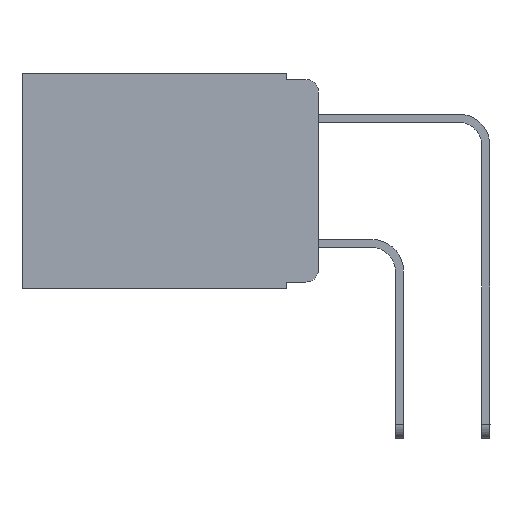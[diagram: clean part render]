
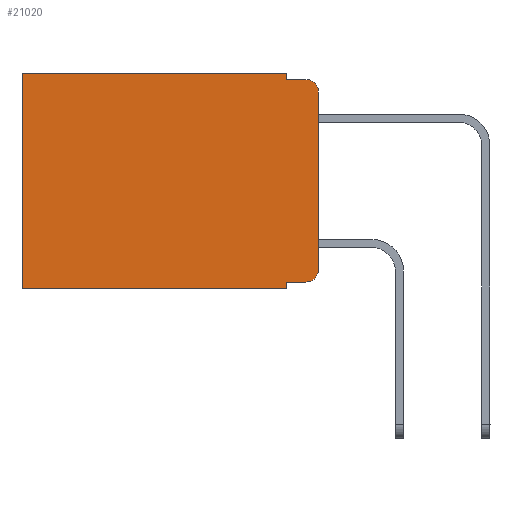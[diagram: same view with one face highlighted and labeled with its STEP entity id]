
A CAD part, left-side view. The second image highlights one B-rep face of the part: STEP entity #21020.
In plain terms, the highlighted planar face has unit normal (-1, 0, 0).
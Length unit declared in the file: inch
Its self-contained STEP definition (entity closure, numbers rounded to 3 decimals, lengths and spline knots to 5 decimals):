
#37 = VECTOR ( 'NONE', #13561, 39.37008 ) ;
#438 = DIRECTION ( 'NONE',  ( 0., 1., 0. ) ) ;
#453 = CARTESIAN_POINT ( 'NONE',  ( 0.298, 0., -0.343 ) ) ;
#503 = ORIENTED_EDGE ( 'NONE', *, *, #20893, .F. ) ;
#535 = CARTESIAN_POINT ( 'NONE',  ( 0.298, 0., 0. ) ) ;
#558 = DIRECTION ( 'NONE',  ( 0., 0., -1. ) ) ;
#646 = DIRECTION ( 'NONE',  ( -1., 0., 0. ) ) ;
#1239 = CARTESIAN_POINT ( 'NONE',  ( 0.298, 0.051, 0. ) ) ;
#1347 = VERTEX_POINT ( 'NONE', #8051 ) ;
#1409 = ORIENTED_EDGE ( 'NONE', *, *, #9598, .F. ) ;
#1495 = CARTESIAN_POINT ( 'NONE',  ( 0.298, 0.02, -0.03 ) ) ;
#1526 = DIRECTION ( 'NONE',  ( 0., 0., -1. ) ) ;
#1839 = AXIS2_PLACEMENT_3D ( 'NONE', #535, #12584, #7223 ) ;
#1972 = CARTESIAN_POINT ( 'NONE',  ( 0.298, 0., 0. ) ) ;
#2070 = PLANE ( 'NONE',  #1839 ) ;
#2104 = EDGE_CURVE ( 'NONE', #11948, #15427, #5297, .T. ) ;
#2612 = VERTEX_POINT ( 'NONE', #21435 ) ;
#3459 = DIRECTION ( 'NONE',  ( 0., -1., 0. ) ) ;
#3470 = ORIENTED_EDGE ( 'NONE', *, *, #9523, .F. ) ;
#3504 = ORIENTED_EDGE ( 'NONE', *, *, #13205, .T. ) ;
#3536 = VECTOR ( 'NONE', #438, 39.37008 ) ;
#3692 = VERTEX_POINT ( 'NONE', #17944 ) ;
#4054 = ORIENTED_EDGE ( 'NONE', *, *, #5171, .F. ) ;
#4130 = CARTESIAN_POINT ( 'NONE',  ( 0.298, 0., -0.03 ) ) ;
#5079 = CARTESIAN_POINT ( 'NONE',  ( 0.298, 0.051, -0.343 ) ) ;
#5171 = EDGE_CURVE ( 'NONE', #1347, #13884, #13077, .T. ) ;
#5297 = CIRCLE ( 'NONE', #17579, 0.02 ) ;
#5930 = CARTESIAN_POINT ( 'NONE',  ( 0.298, 0.02, -0.01 ) ) ;
#6796 = LINE ( 'NONE', #1972, #3536 ) ;
#6936 = VECTOR ( 'NONE', #558, 39.37008 ) ;
#7045 = ORIENTED_EDGE ( 'NONE', *, *, #19641, .F. ) ;
#7223 = DIRECTION ( 'NONE',  ( 0., 0., -1. ) ) ;
#7253 = LINE ( 'NONE', #20646, #6936 ) ;
#7352 = DIRECTION ( 'NONE',  ( 0., 0., -1. ) ) ;
#7904 = VERTEX_POINT ( 'NONE', #18206 ) ;
#8051 = CARTESIAN_POINT ( 'NONE',  ( 0.298, 0.051, -0.333 ) ) ;
#8715 = VERTEX_POINT ( 'NONE', #4130 ) ;
#9043 = EDGE_CURVE ( 'NONE', #1347, #11948, #18480, .T. ) ;
#9523 = EDGE_CURVE ( 'NONE', #8715, #15427, #7253, .T. ) ;
#9598 = EDGE_CURVE ( 'NONE', #13884, #11979, #20423, .T. ) ;
#9652 = VERTEX_POINT ( 'NONE', #5930 ) ;
#10512 = CIRCLE ( 'NONE', #15761, 0.02 ) ;
#11040 = EDGE_CURVE ( 'NONE', #2612, #11979, #18216, .T. ) ;
#11823 = LINE ( 'NONE', #15349, #17975 ) ;
#11948 = VERTEX_POINT ( 'NONE', #15339 ) ;
#11979 = VERTEX_POINT ( 'NONE', #14233 ) ;
#12195 = VECTOR ( 'NONE', #1526, 39.37008 ) ;
#12303 = ORIENTED_EDGE ( 'NONE', *, *, #11040, .T. ) ;
#12584 = DIRECTION ( 'NONE',  ( 1., 0., 0. ) ) ;
#12633 = CARTESIAN_POINT ( 'NONE',  ( 0.298, 0., -0.313 ) ) ;
#13077 = LINE ( 'NONE', #1239, #15934 ) ;
#13205 = EDGE_CURVE ( 'NONE', #3692, #2612, #6796, .T. ) ;
#13340 = DIRECTION ( 'NONE',  ( -1., 0., 0. ) ) ;
#13561 = DIRECTION ( 'NONE',  ( 0., -1., 0. ) ) ;
#13643 = CARTESIAN_POINT ( 'NONE',  ( 0.298, 0.051, -0.333 ) ) ;
#13884 = VERTEX_POINT ( 'NONE', #5079 ) ;
#14233 = CARTESIAN_POINT ( 'NONE',  ( 0.298, 0.473, -0.343 ) ) ;
#14464 = ORIENTED_EDGE ( 'NONE', *, *, #9043, .T. ) ;
#14468 = EDGE_LOOP ( 'NONE', ( #3470, #16345, #7045, #503, #3504, #12303, #1409, #4054, #14464, #18204 ) ) ;
#15225 = CARTESIAN_POINT ( 'NONE',  ( 0.298, 0.051, -0.01 ) ) ;
#15339 = CARTESIAN_POINT ( 'NONE',  ( 0.298, 0.02, -0.333 ) ) ;
#15349 = CARTESIAN_POINT ( 'NONE',  ( 0.298, 0.051, 0. ) ) ;
#15427 = VERTEX_POINT ( 'NONE', #12633 ) ;
#15574 = FACE_OUTER_BOUND ( 'NONE', #14468, .T. ) ;
#15724 = VECTOR ( 'NONE', #17141, 39.37008 ) ;
#15761 = AXIS2_PLACEMENT_3D ( 'NONE', #1495, #13340, #19013 ) ;
#15934 = VECTOR ( 'NONE', #21336, 39.37008 ) ;
#16345 = ORIENTED_EDGE ( 'NONE', *, *, #18328, .T. ) ;
#17141 = DIRECTION ( 'NONE',  ( 0., 1., 0. ) ) ;
#17339 = CARTESIAN_POINT ( 'NONE',  ( 0.298, 0.02, -0.313 ) ) ;
#17579 = AXIS2_PLACEMENT_3D ( 'NONE', #17339, #646, #7352 ) ;
#17944 = CARTESIAN_POINT ( 'NONE',  ( 0.298, 0.051, 0. ) ) ;
#17975 = VECTOR ( 'NONE', #21602, 39.37008 ) ;
#18204 = ORIENTED_EDGE ( 'NONE', *, *, #2104, .T. ) ;
#18206 = CARTESIAN_POINT ( 'NONE',  ( 0.298, 0.051, -0.01 ) ) ;
#18216 = LINE ( 'NONE', #19964, #12195 ) ;
#18328 = EDGE_CURVE ( 'NONE', #8715, #9652, #10512, .T. ) ;
#18480 = LINE ( 'NONE', #13643, #19890 ) ;
#19013 = DIRECTION ( 'NONE',  ( 0., 0., -1. ) ) ;
#19058 = LINE ( 'NONE', #15225, #37 ) ;
#19641 = EDGE_CURVE ( 'NONE', #7904, #9652, #19058, .T. ) ;
#19890 = VECTOR ( 'NONE', #3459, 39.37008 ) ;
#19964 = CARTESIAN_POINT ( 'NONE',  ( 0.298, 0.473, 0. ) ) ;
#20423 = LINE ( 'NONE', #453, #15724 ) ;
#20646 = CARTESIAN_POINT ( 'NONE',  ( 0.298, 0., 0. ) ) ;
#20893 = EDGE_CURVE ( 'NONE', #3692, #7904, #11823, .T. ) ;
#21020 = ADVANCED_FACE ( 'NONE', ( #15574 ), #2070, .F. ) ;
#21336 = DIRECTION ( 'NONE',  ( 0., 0., -1. ) ) ;
#21435 = CARTESIAN_POINT ( 'NONE',  ( 0.298, 0.473, 0. ) ) ;
#21602 = DIRECTION ( 'NONE',  ( 0., 0., -1. ) ) ;
